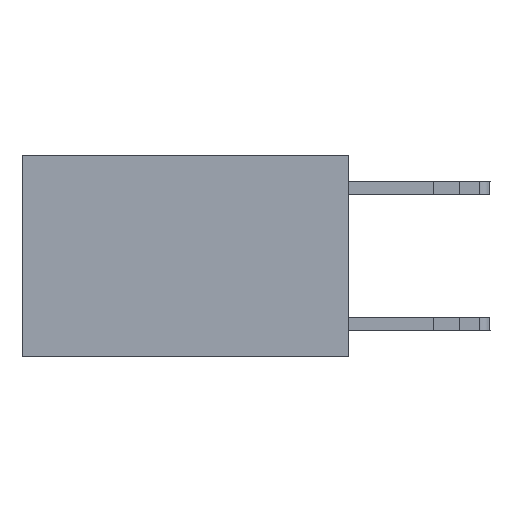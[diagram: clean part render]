
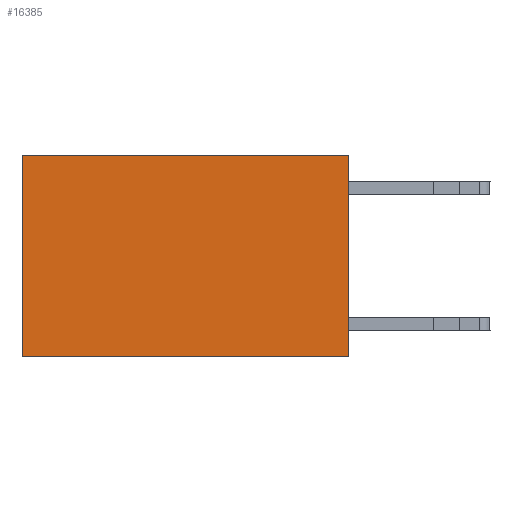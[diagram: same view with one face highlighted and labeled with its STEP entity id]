
A CAD part, left-side view. The second image highlights one B-rep face of the part: STEP entity #16385.
In plain terms, the highlighted planar face has unit normal (-1, 0, 0).
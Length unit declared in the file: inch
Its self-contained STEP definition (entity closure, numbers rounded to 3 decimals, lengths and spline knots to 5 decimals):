
#82 = DIRECTION ( 'NONE',  ( 0., 1., 0. ) ) ;
#1800 = DIRECTION ( 'NONE',  ( 0., 0., -1. ) ) ;
#1992 = EDGE_CURVE ( 'NONE', #9523, #26141, #19942, .T. ) ;
#3984 = EDGE_LOOP ( 'NONE', ( #13746, #12566, #13878, #15275 ) ) ;
#4268 = PLANE ( 'NONE',  #9473 ) ;
#4358 = VERTEX_POINT ( 'NONE', #20495 ) ;
#5650 = CARTESIAN_POINT ( 'NONE',  ( 0.2625, 0.6, 0. ) ) ;
#6158 = CARTESIAN_POINT ( 'NONE',  ( 0.2625, 0., -0.37 ) ) ;
#6293 = CARTESIAN_POINT ( 'NONE',  ( 0.2625, 0., -0.37 ) ) ;
#6362 = LINE ( 'NONE', #19439, #20010 ) ;
#7943 = VECTOR ( 'NONE', #26668, 39.37008 ) ;
#8491 = FACE_OUTER_BOUND ( 'NONE', #3984, .T. ) ;
#8858 = VECTOR ( 'NONE', #14096, 39.37008 ) ;
#9473 = AXIS2_PLACEMENT_3D ( 'NONE', #10818, #19516, #1800 ) ;
#9523 = VERTEX_POINT ( 'NONE', #6158 ) ;
#10818 = CARTESIAN_POINT ( 'NONE',  ( 0.2625, 0., 0. ) ) ;
#11038 = EDGE_CURVE ( 'NONE', #4358, #26141, #18743, .T. ) ;
#11785 = EDGE_CURVE ( 'NONE', #16216, #4358, #25171, .T. ) ;
#12566 = ORIENTED_EDGE ( 'NONE', *, *, #1992, .F. ) ;
#13746 = ORIENTED_EDGE ( 'NONE', *, *, #11038, .T. ) ;
#13878 = ORIENTED_EDGE ( 'NONE', *, *, #21711, .F. ) ;
#14096 = DIRECTION ( 'NONE',  ( 0., 0., -1. ) ) ;
#15275 = ORIENTED_EDGE ( 'NONE', *, *, #11785, .T. ) ;
#15639 = CARTESIAN_POINT ( 'NONE',  ( 0.2625, 0., 0. ) ) ;
#16216 = VERTEX_POINT ( 'NONE', #25472 ) ;
#16385 = ADVANCED_FACE ( 'NONE', ( #8491 ), #4268, .F. ) ;
#17897 = CARTESIAN_POINT ( 'NONE',  ( 0.2625, 0.6, -0.37 ) ) ;
#18743 = LINE ( 'NONE', #5650, #8858 ) ;
#19439 = CARTESIAN_POINT ( 'NONE',  ( 0.2625, 0., 0. ) ) ;
#19516 = DIRECTION ( 'NONE',  ( 1., 0., 0. ) ) ;
#19942 = LINE ( 'NONE', #6293, #28523 ) ;
#20010 = VECTOR ( 'NONE', #26128, 39.37008 ) ;
#20495 = CARTESIAN_POINT ( 'NONE',  ( 0.2625, 0.6, 0. ) ) ;
#21711 = EDGE_CURVE ( 'NONE', #16216, #9523, #6362, .T. ) ;
#25171 = LINE ( 'NONE', #15639, #7943 ) ;
#25472 = CARTESIAN_POINT ( 'NONE',  ( 0.2625, 0., 0. ) ) ;
#26128 = DIRECTION ( 'NONE',  ( 0., 0., -1. ) ) ;
#26141 = VERTEX_POINT ( 'NONE', #17897 ) ;
#26668 = DIRECTION ( 'NONE',  ( 0., 1., 0. ) ) ;
#28523 = VECTOR ( 'NONE', #82, 39.37008 ) ;
